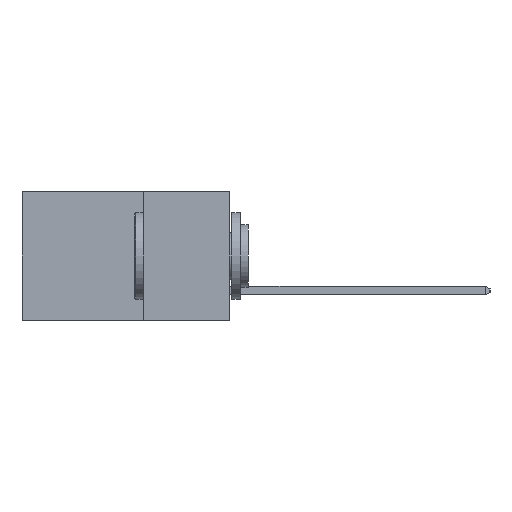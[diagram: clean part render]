
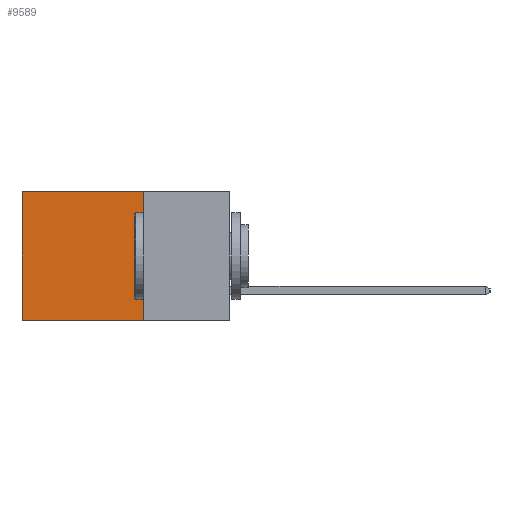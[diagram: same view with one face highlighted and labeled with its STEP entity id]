
A CAD part, left-side view. The second image highlights one B-rep face of the part: STEP entity #9589.
In plain terms, the highlighted planar face has unit normal (-1, 0, 0).
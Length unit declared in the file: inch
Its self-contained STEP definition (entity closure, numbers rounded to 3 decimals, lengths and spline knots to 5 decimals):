
#38 = EDGE_CURVE ( 'NONE', #12528, #12338, #7708, .T. ) ;
#113 = VERTEX_POINT ( 'NONE', #6133 ) ;
#270 = CARTESIAN_POINT ( 'NONE',  ( 0.298, 0.25, 0. ) ) ;
#322 = DIRECTION ( 'NONE',  ( 0., 0., -1. ) ) ;
#429 = DIRECTION ( 'NONE',  ( 0., 1., 0. ) ) ;
#433 = CARTESIAN_POINT ( 'NONE',  ( 0.298, 0.6, 0. ) ) ;
#805 = LINE ( 'NONE', #2535, #11004 ) ;
#1171 = FACE_OUTER_BOUND ( 'NONE', #8645, .T. ) ;
#1433 = DIRECTION ( 'NONE',  ( 0., 0., -1. ) ) ;
#1565 = CARTESIAN_POINT ( 'NONE',  ( 0.298, 0.25, 0. ) ) ;
#2015 = CARTESIAN_POINT ( 'NONE',  ( 0.298, 0.25, 0. ) ) ;
#2535 = CARTESIAN_POINT ( 'NONE',  ( 0.298, 0.25, -0.37 ) ) ;
#2708 = CARTESIAN_POINT ( 'NONE',  ( 0.298, 0.25, 0. ) ) ;
#3135 = PLANE ( 'NONE',  #11164 ) ;
#3440 = DIRECTION ( 'NONE',  ( 0., 1., 0. ) ) ;
#3444 = CARTESIAN_POINT ( 'NONE',  ( 0.298, 0.6, 0. ) ) ;
#4130 = VECTOR ( 'NONE', #1433, 39.37008 ) ;
#4449 = LINE ( 'NONE', #270, #11670 ) ;
#5052 = VECTOR ( 'NONE', #3440, 39.37008 ) ;
#6111 = ORIENTED_EDGE ( 'NONE', *, *, #6612, .T. ) ;
#6133 = CARTESIAN_POINT ( 'NONE',  ( 0.298, 0.25, -0.37 ) ) ;
#6201 = DIRECTION ( 'NONE',  ( 0., 0., -1. ) ) ;
#6612 = EDGE_CURVE ( 'NONE', #12338, #8222, #9590, .T. ) ;
#7114 = ORIENTED_EDGE ( 'NONE', *, *, #11165, .F. ) ;
#7708 = LINE ( 'NONE', #2708, #5052 ) ;
#7829 = ORIENTED_EDGE ( 'NONE', *, *, #38, .T. ) ;
#8222 = VERTEX_POINT ( 'NONE', #9011 ) ;
#8645 = EDGE_LOOP ( 'NONE', ( #6111, #7114, #9546, #7829 ) ) ;
#9011 = CARTESIAN_POINT ( 'NONE',  ( 0.298, 0.6, -0.37 ) ) ;
#9546 = ORIENTED_EDGE ( 'NONE', *, *, #11673, .F. ) ;
#9589 = ADVANCED_FACE ( 'NONE', ( #1171 ), #3135, .F. ) ;
#9590 = LINE ( 'NONE', #433, #4130 ) ;
#11004 = VECTOR ( 'NONE', #429, 39.37008 ) ;
#11164 = AXIS2_PLACEMENT_3D ( 'NONE', #2015, #11718, #6201 ) ;
#11165 = EDGE_CURVE ( 'NONE', #113, #8222, #805, .T. ) ;
#11670 = VECTOR ( 'NONE', #322, 39.37008 ) ;
#11673 = EDGE_CURVE ( 'NONE', #12528, #113, #4449, .T. ) ;
#11718 = DIRECTION ( 'NONE',  ( 1., 0., 0. ) ) ;
#12338 = VERTEX_POINT ( 'NONE', #3444 ) ;
#12528 = VERTEX_POINT ( 'NONE', #1565 ) ;
